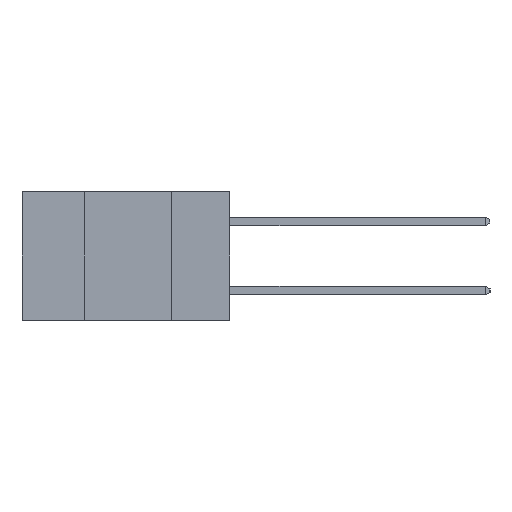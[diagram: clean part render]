
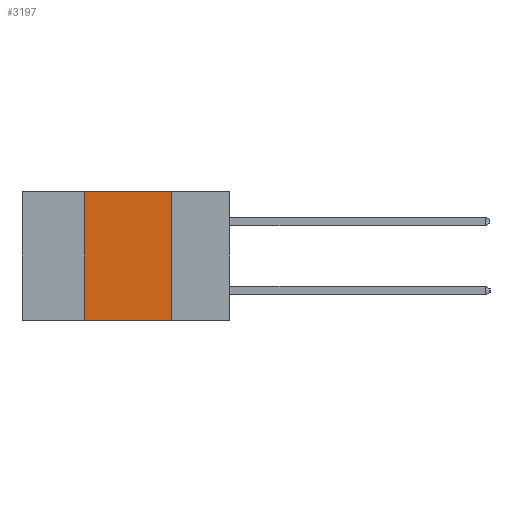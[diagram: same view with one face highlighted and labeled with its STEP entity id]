
A CAD part, left-side view. The second image highlights one B-rep face of the part: STEP entity #3197.
In plain terms, the highlighted planar face has unit normal (-1, 0, 0).
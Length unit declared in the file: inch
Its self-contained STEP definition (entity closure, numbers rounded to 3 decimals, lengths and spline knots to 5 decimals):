
#612 = LINE ( 'NONE', #12545, #9576 ) ;
#1112 = DIRECTION ( 'NONE',  ( 0., 0., 1. ) ) ;
#1309 = LINE ( 'NONE', #2498, #4055 ) ;
#1324 = CARTESIAN_POINT ( 'NONE',  ( 0., 0.6, 0. ) ) ;
#1635 = CARTESIAN_POINT ( 'NONE',  ( 0., 0.17, 0. ) ) ;
#1788 = CARTESIAN_POINT ( 'NONE',  ( 0., 0.42, -0.37 ) ) ;
#1805 = EDGE_CURVE ( 'NONE', #13872, #14175, #1309, .T. ) ;
#1843 = DIRECTION ( 'NONE',  ( 0., -1., 0. ) ) ;
#1864 = ORIENTED_EDGE ( 'NONE', *, *, #1805, .T. ) ;
#2498 = CARTESIAN_POINT ( 'NONE',  ( 0., 0.6, -0.37 ) ) ;
#2980 = EDGE_CURVE ( 'NONE', #14528, #14175, #10908, .T. ) ;
#3197 = ADVANCED_FACE ( 'NONE', ( #10368 ), #8592, .F. ) ;
#3198 = CARTESIAN_POINT ( 'NONE',  ( 0., 0.17, -0.37 ) ) ;
#3917 = VECTOR ( 'NONE', #1112, 39.37008 ) ;
#3965 = EDGE_LOOP ( 'NONE', ( #10410, #7780, #13669, #1864 ) ) ;
#4055 = VECTOR ( 'NONE', #1843, 39.37008 ) ;
#4503 = DIRECTION ( 'NONE',  ( 0., 0., -1. ) ) ;
#4694 = DIRECTION ( 'NONE',  ( 0., 0., -1. ) ) ;
#5198 = CARTESIAN_POINT ( 'NONE',  ( 0., 0.17, -0.37 ) ) ;
#7158 = VERTEX_POINT ( 'NONE', #12826 ) ;
#7466 = LINE ( 'NONE', #1788, #3917 ) ;
#7729 = CARTESIAN_POINT ( 'NONE',  ( 0., 0.42, -0.37 ) ) ;
#7780 = ORIENTED_EDGE ( 'NONE', *, *, #8064, .F. ) ;
#7851 = EDGE_CURVE ( 'NONE', #13872, #7158, #7466, .T. ) ;
#8064 = EDGE_CURVE ( 'NONE', #7158, #14528, #612, .T. ) ;
#8592 = PLANE ( 'NONE',  #11917 ) ;
#9576 = VECTOR ( 'NONE', #12565, 39.37008 ) ;
#10368 = FACE_OUTER_BOUND ( 'NONE', #3965, .T. ) ;
#10410 = ORIENTED_EDGE ( 'NONE', *, *, #2980, .F. ) ;
#10908 = LINE ( 'NONE', #3198, #13132 ) ;
#11215 = DIRECTION ( 'NONE',  ( 1., 0., 0. ) ) ;
#11917 = AXIS2_PLACEMENT_3D ( 'NONE', #1324, #11215, #4503 ) ;
#12545 = CARTESIAN_POINT ( 'NONE',  ( 0., 0.6, 0. ) ) ;
#12565 = DIRECTION ( 'NONE',  ( 0., -1., 0. ) ) ;
#12826 = CARTESIAN_POINT ( 'NONE',  ( 0., 0.42, 0. ) ) ;
#13132 = VECTOR ( 'NONE', #4694, 39.37008 ) ;
#13669 = ORIENTED_EDGE ( 'NONE', *, *, #7851, .F. ) ;
#13872 = VERTEX_POINT ( 'NONE', #7729 ) ;
#14175 = VERTEX_POINT ( 'NONE', #5198 ) ;
#14528 = VERTEX_POINT ( 'NONE', #1635 ) ;
